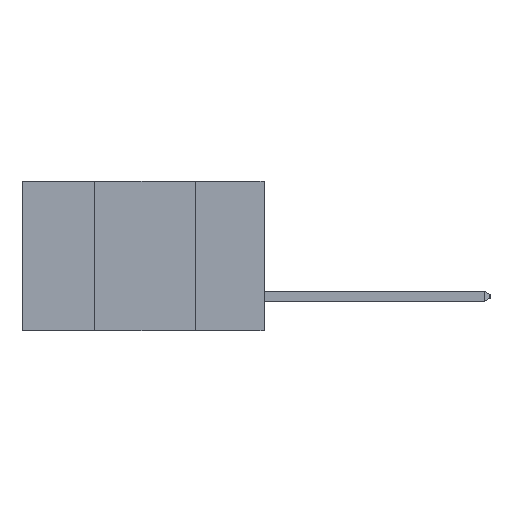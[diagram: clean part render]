
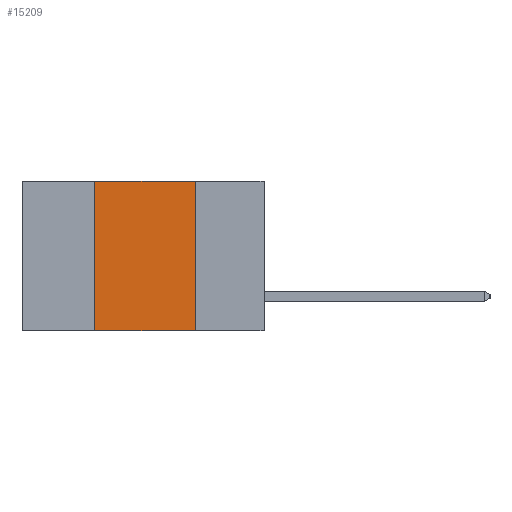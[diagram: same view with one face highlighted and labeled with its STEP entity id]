
A CAD part, left-side view. The second image highlights one B-rep face of the part: STEP entity #15209.
In plain terms, the highlighted planar face has unit normal (-1, 0, 0).
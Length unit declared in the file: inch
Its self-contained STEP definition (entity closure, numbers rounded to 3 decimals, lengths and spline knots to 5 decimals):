
#1051 = CARTESIAN_POINT ( 'NONE',  ( 0., 0.17, -0.37 ) ) ;
#1218 = CARTESIAN_POINT ( 'NONE',  ( 0., 0.6, 0. ) ) ;
#1315 = CARTESIAN_POINT ( 'NONE',  ( 0., 0.42, 0. ) ) ;
#1457 = DIRECTION ( 'NONE',  ( 0., -1., 0. ) ) ;
#1783 = LINE ( 'NONE', #17226, #12140 ) ;
#1907 = CARTESIAN_POINT ( 'NONE',  ( 0., 0.6, -0.37 ) ) ;
#3369 = DIRECTION ( 'NONE',  ( 0., -1., 0. ) ) ;
#4138 = PLANE ( 'NONE',  #10629 ) ;
#5230 = ORIENTED_EDGE ( 'NONE', *, *, #15390, .F. ) ;
#5431 = VERTEX_POINT ( 'NONE', #6858 ) ;
#5441 = DIRECTION ( 'NONE',  ( 1., 0., 0. ) ) ;
#5523 = ORIENTED_EDGE ( 'NONE', *, *, #16021, .F. ) ;
#6312 = ORIENTED_EDGE ( 'NONE', *, *, #8991, .F. ) ;
#6858 = CARTESIAN_POINT ( 'NONE',  ( 0., 0.17, 0. ) ) ;
#7353 = LINE ( 'NONE', #14996, #13515 ) ;
#7517 = VECTOR ( 'NONE', #3369, 39.37008 ) ;
#7982 = CARTESIAN_POINT ( 'NONE',  ( 0., 0.42, -0.37 ) ) ;
#8488 = CARTESIAN_POINT ( 'NONE',  ( 0., 0.42, 0. ) ) ;
#8991 = EDGE_CURVE ( 'NONE', #5431, #13650, #7353, .T. ) ;
#9095 = EDGE_LOOP ( 'NONE', ( #6312, #5523, #5230, #16631 ) ) ;
#9711 = FACE_OUTER_BOUND ( 'NONE', #9095, .T. ) ;
#10113 = VERTEX_POINT ( 'NONE', #7982 ) ;
#10629 = AXIS2_PLACEMENT_3D ( 'NONE', #1218, #5441, #14594 ) ;
#12140 = VECTOR ( 'NONE', #1457, 39.37008 ) ;
#13515 = VECTOR ( 'NONE', #16248, 39.37008 ) ;
#13650 = VERTEX_POINT ( 'NONE', #1051 ) ;
#13712 = LINE ( 'NONE', #8488, #16639 ) ;
#14470 = LINE ( 'NONE', #1907, #7517 ) ;
#14594 = DIRECTION ( 'NONE',  ( 0., 0., -1. ) ) ;
#14862 = DIRECTION ( 'NONE',  ( 0., 0., 1. ) ) ;
#14996 = CARTESIAN_POINT ( 'NONE',  ( 0., 0.17, 0. ) ) ;
#15209 = ADVANCED_FACE ( 'NONE', ( #9711 ), #4138, .F. ) ;
#15390 = EDGE_CURVE ( 'NONE', #10113, #16500, #13712, .T. ) ;
#16021 = EDGE_CURVE ( 'NONE', #16500, #5431, #1783, .T. ) ;
#16225 = EDGE_CURVE ( 'NONE', #10113, #13650, #14470, .T. ) ;
#16248 = DIRECTION ( 'NONE',  ( 0., 0., -1. ) ) ;
#16500 = VERTEX_POINT ( 'NONE', #1315 ) ;
#16631 = ORIENTED_EDGE ( 'NONE', *, *, #16225, .T. ) ;
#16639 = VECTOR ( 'NONE', #14862, 39.37008 ) ;
#17226 = CARTESIAN_POINT ( 'NONE',  ( 0., 0.6, 0. ) ) ;
